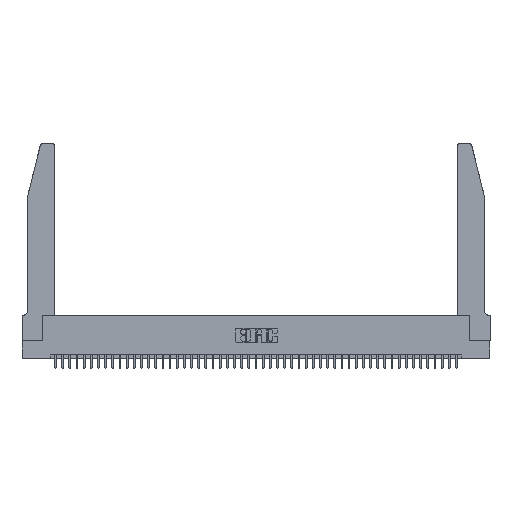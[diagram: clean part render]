
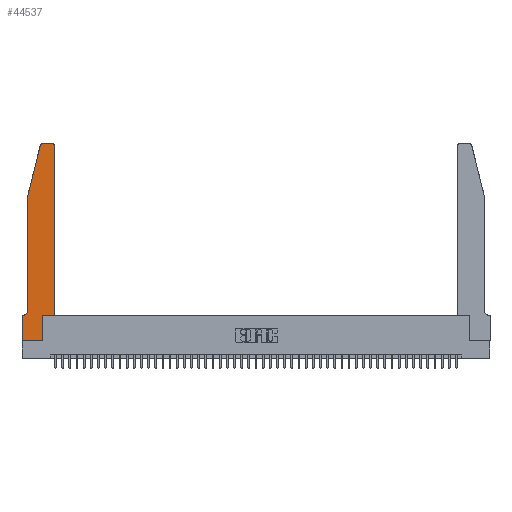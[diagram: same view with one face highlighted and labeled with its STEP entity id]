
A CAD part, top view. The second image highlights one B-rep face of the part: STEP entity #44537.
In plain terms, the highlighted planar face has unit normal (0, 0, 1).
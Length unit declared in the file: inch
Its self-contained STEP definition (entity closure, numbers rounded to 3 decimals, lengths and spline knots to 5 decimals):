
#9 = VERTEX_POINT ( 'NONE', #7081 ) ;
#771 = EDGE_CURVE ( 'NONE', #9, #26985, #35800, .T. ) ;
#814 = LINE ( 'NONE', #45268, #17044 ) ;
#2121 = ORIENTED_EDGE ( 'NONE', *, *, #2858, .T. ) ;
#2858 = EDGE_CURVE ( 'NONE', #32288, #32094, #7595, .T. ) ;
#2892 = ORIENTED_EDGE ( 'NONE', *, *, #27732, .T. ) ;
#4550 = EDGE_CURVE ( 'NONE', #21497, #18745, #18302, .T. ) ;
#4992 = VERTEX_POINT ( 'NONE', #15553 ) ;
#5186 = CARTESIAN_POINT ( 'NONE',  ( 0.0055, 0.42, 0.37 ) ) ;
#5288 = EDGE_CURVE ( 'NONE', #24219, #46663, #35521, .T. ) ;
#5658 = CARTESIAN_POINT ( 'NONE',  ( 0.2865, 0., 0.37 ) ) ;
#5708 = ORIENTED_EDGE ( 'NONE', *, *, #28783, .T. ) ;
#5984 = CARTESIAN_POINT ( 'NONE',  ( 0.4505, 0.35, 0.37 ) ) ;
#6293 = CARTESIAN_POINT ( 'NONE',  ( 0.25487, 2.72718, 0.37 ) ) ;
#6928 = AXIS2_PLACEMENT_3D ( 'NONE', #14979, #22023, #18642 ) ;
#7081 = CARTESIAN_POINT ( 'NONE',  ( 0.0055, 0.35, 0.37 ) ) ;
#7175 = DIRECTION ( 'NONE',  ( 0., 1., 0. ) ) ;
#7413 = LINE ( 'NONE', #31159, #33165 ) ;
#7537 = AXIS2_PLACEMENT_3D ( 'NONE', #5186, #10364, #23761 ) ;
#7595 = CIRCLE ( 'NONE', #45481, 0.03 ) ;
#10039 = DIRECTION ( 'NONE',  ( -0.239, -0.971, 0. ) ) ;
#10364 = DIRECTION ( 'NONE',  ( 0., 0., -1. ) ) ;
#10656 = EDGE_CURVE ( 'NONE', #4992, #25037, #32718, .T. ) ;
#12368 = VECTOR ( 'NONE', #25575, 39.37008 ) ;
#12565 = DIRECTION ( 'NONE',  ( 0., 0., 1. ) ) ;
#12584 = VERTEX_POINT ( 'NONE', #39368 ) ;
#12741 = ORIENTED_EDGE ( 'NONE', *, *, #17832, .T. ) ;
#13211 = DIRECTION ( 'NONE',  ( 1., 0., 0. ) ) ;
#14008 = EDGE_CURVE ( 'NONE', #26985, #4992, #7413, .T. ) ;
#14979 = CARTESIAN_POINT ( 'NONE',  ( 0.284, 2.72, 0.37 ) ) ;
#15387 = ORIENTED_EDGE ( 'NONE', *, *, #39638, .T. ) ;
#15553 = CARTESIAN_POINT ( 'NONE',  ( 0., 0., 0.37 ) ) ;
#17044 = VECTOR ( 'NONE', #40786, 39.37008 ) ;
#17832 = EDGE_CURVE ( 'NONE', #29155, #9, #24276, .T. ) ;
#17895 = CARTESIAN_POINT ( 'NONE',  ( 0.2865, 0.35, 0.37 ) ) ;
#18302 = LINE ( 'NONE', #32093, #36611 ) ;
#18642 = DIRECTION ( 'NONE',  ( 1., 0., 0. ) ) ;
#18745 = VERTEX_POINT ( 'NONE', #5984 ) ;
#19364 = DIRECTION ( 'NONE',  ( 0., 0., 1. ) ) ;
#20368 = CARTESIAN_POINT ( 'NONE',  ( 0.4205, 2.72, 0.37 ) ) ;
#21117 = CIRCLE ( 'NONE', #6928, 0.03 ) ;
#21145 = LINE ( 'NONE', #17895, #26248 ) ;
#21497 = VERTEX_POINT ( 'NONE', #46483 ) ;
#22023 = DIRECTION ( 'NONE',  ( 0., 0., 1. ) ) ;
#22989 = CARTESIAN_POINT ( 'NONE',  ( 0.0755, 2., 0.37 ) ) ;
#23284 = CARTESIAN_POINT ( 'NONE',  ( 0.0755, 0.42, 0.37 ) ) ;
#23429 = CARTESIAN_POINT ( 'NONE',  ( 0., 0.35, 0.37 ) ) ;
#23761 = DIRECTION ( 'NONE',  ( -1., 0., 0. ) ) ;
#23940 = EDGE_CURVE ( 'NONE', #32094, #12584, #814, .T. ) ;
#24219 = VERTEX_POINT ( 'NONE', #6293 ) ;
#24276 = CIRCLE ( 'NONE', #7537, 0.07 ) ;
#24732 = ORIENTED_EDGE ( 'NONE', *, *, #23940, .T. ) ;
#25037 = VERTEX_POINT ( 'NONE', #5658 ) ;
#25408 = VECTOR ( 'NONE', #44568, 39.37008 ) ;
#25575 = DIRECTION ( 'NONE',  ( -1., 0., 0. ) ) ;
#25771 = CARTESIAN_POINT ( 'NONE',  ( 0.0755, 2., 0.37 ) ) ;
#26248 = VECTOR ( 'NONE', #7175, 39.37008 ) ;
#26985 = VERTEX_POINT ( 'NONE', #23429 ) ;
#27444 = VECTOR ( 'NONE', #37127, 39.37008 ) ;
#27458 = CARTESIAN_POINT ( 'NONE',  ( 0.0755, 2., 0.37 ) ) ;
#27732 = EDGE_CURVE ( 'NONE', #46663, #29155, #41157, .T. ) ;
#28151 = AXIS2_PLACEMENT_3D ( 'NONE', #36827, #12565, #37302 ) ;
#28783 = EDGE_CURVE ( 'NONE', #12584, #24219, #21117, .T. ) ;
#28956 = EDGE_LOOP ( 'NONE', ( #24732, #5708, #35022, #2892, #12741, #29393, #29791, #45854, #15387, #34180, #30940, #2121 ) ) ;
#29155 = VERTEX_POINT ( 'NONE', #23284 ) ;
#29294 = CARTESIAN_POINT ( 'NONE',  ( 0., 0., 0.37 ) ) ;
#29296 = VECTOR ( 'NONE', #36619, 39.37008 ) ;
#29393 = ORIENTED_EDGE ( 'NONE', *, *, #771, .T. ) ;
#29791 = ORIENTED_EDGE ( 'NONE', *, *, #14008, .T. ) ;
#29837 = CARTESIAN_POINT ( 'NONE',  ( 0.4205, 2.75, 0.37 ) ) ;
#29934 = VECTOR ( 'NONE', #10039, 39.37008 ) ;
#30940 = ORIENTED_EDGE ( 'NONE', *, *, #42952, .T. ) ;
#31159 = CARTESIAN_POINT ( 'NONE',  ( 0., 0., 0.37 ) ) ;
#32093 = CARTESIAN_POINT ( 'NONE',  ( 0.4505, 0.35, 0.37 ) ) ;
#32094 = VERTEX_POINT ( 'NONE', #29837 ) ;
#32288 = VERTEX_POINT ( 'NONE', #38425 ) ;
#32718 = LINE ( 'NONE', #29294, #29296 ) ;
#33165 = VECTOR ( 'NONE', #41537, 39.37008 ) ;
#33533 = CARTESIAN_POINT ( 'NONE',  ( 0.4505, 0.35, 0.37 ) ) ;
#33611 = PLANE ( 'NONE',  #28151 ) ;
#34180 = ORIENTED_EDGE ( 'NONE', *, *, #4550, .T. ) ;
#34741 = FACE_OUTER_BOUND ( 'NONE', #28956, .T. ) ;
#35022 = ORIENTED_EDGE ( 'NONE', *, *, #5288, .T. ) ;
#35521 = LINE ( 'NONE', #27458, #29934 ) ;
#35749 = DIRECTION ( 'NONE',  ( 1., 0., 0. ) ) ;
#35800 = LINE ( 'NONE', #43663, #12368 ) ;
#36611 = VECTOR ( 'NONE', #35749, 39.37008 ) ;
#36619 = DIRECTION ( 'NONE',  ( 1., 0., 0. ) ) ;
#36827 = CARTESIAN_POINT ( 'NONE',  ( 0., 0.35, 0.37 ) ) ;
#37127 = DIRECTION ( 'NONE',  ( 0., -1., 0. ) ) ;
#37302 = DIRECTION ( 'NONE',  ( 1., 0., 0. ) ) ;
#38425 = CARTESIAN_POINT ( 'NONE',  ( 0.4505, 2.72, 0.37 ) ) ;
#39368 = CARTESIAN_POINT ( 'NONE',  ( 0.284, 2.75, 0.37 ) ) ;
#39638 = EDGE_CURVE ( 'NONE', #25037, #21497, #21145, .T. ) ;
#40786 = DIRECTION ( 'NONE',  ( -1., 0., 0. ) ) ;
#41157 = LINE ( 'NONE', #25771, #27444 ) ;
#41537 = DIRECTION ( 'NONE',  ( 0., -1., 0. ) ) ;
#42952 = EDGE_CURVE ( 'NONE', #18745, #32288, #47189, .T. ) ;
#43663 = CARTESIAN_POINT ( 'NONE',  ( 0.0755, 0.35, 0.37 ) ) ;
#44537 = ADVANCED_FACE ( 'NONE', ( #34741 ), #33611, .T. ) ;
#44568 = DIRECTION ( 'NONE',  ( 0., 1., 0. ) ) ;
#45268 = CARTESIAN_POINT ( 'NONE',  ( 0.2605, 2.75, 0.37 ) ) ;
#45481 = AXIS2_PLACEMENT_3D ( 'NONE', #20368, #19364, #13211 ) ;
#45854 = ORIENTED_EDGE ( 'NONE', *, *, #10656, .T. ) ;
#46483 = CARTESIAN_POINT ( 'NONE',  ( 0.2865, 0.35, 0.37 ) ) ;
#46663 = VERTEX_POINT ( 'NONE', #22989 ) ;
#47189 = LINE ( 'NONE', #33533, #25408 ) ;
